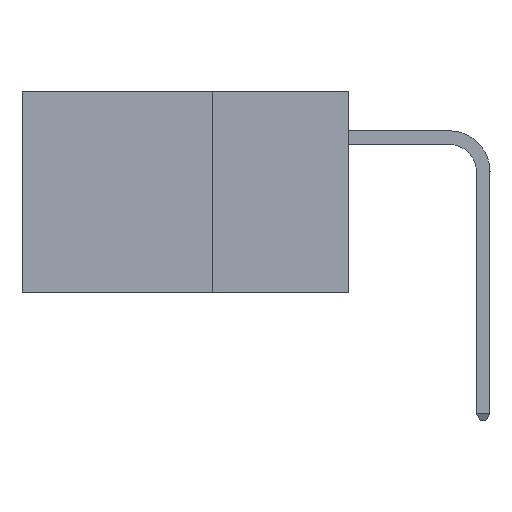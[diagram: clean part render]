
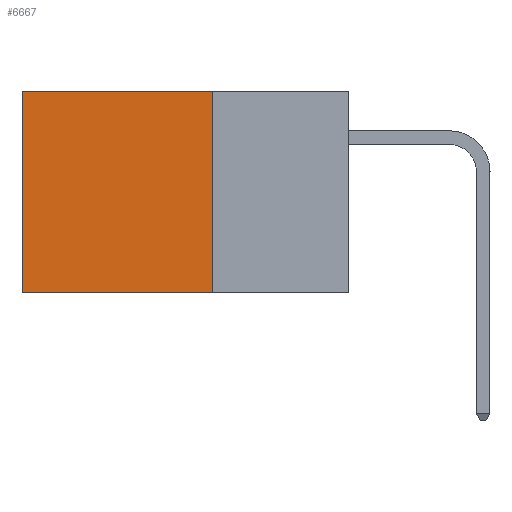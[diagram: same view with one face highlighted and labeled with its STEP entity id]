
A CAD part, left-side view. The second image highlights one B-rep face of the part: STEP entity #6667.
In plain terms, the highlighted planar face has unit normal (-1, 0, 0).
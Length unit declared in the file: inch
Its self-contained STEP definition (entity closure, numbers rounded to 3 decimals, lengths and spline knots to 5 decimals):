
#29 = LINE ( 'NONE', #6393, #11558 ) ;
#331 = VERTEX_POINT ( 'NONE', #14017 ) ;
#605 = VERTEX_POINT ( 'NONE', #11460 ) ;
#2172 = ORIENTED_EDGE ( 'NONE', *, *, #9008, .T. ) ;
#2841 = FACE_OUTER_BOUND ( 'NONE', #14357, .T. ) ;
#3492 = VERTEX_POINT ( 'NONE', #11173 ) ;
#3546 = CARTESIAN_POINT ( 'NONE',  ( 0.2875, 0.6, 0. ) ) ;
#3996 = VERTEX_POINT ( 'NONE', #9984 ) ;
#4261 = VECTOR ( 'NONE', #9499, 39.37008 ) ;
#4561 = VECTOR ( 'NONE', #11154, 39.37008 ) ;
#4612 = LINE ( 'NONE', #8438, #4261 ) ;
#4758 = DIRECTION ( 'NONE',  ( 0., 1., 0. ) ) ;
#5315 = DIRECTION ( 'NONE',  ( 0., 0., -1. ) ) ;
#5615 = VECTOR ( 'NONE', #4758, 39.37008 ) ;
#5926 = CARTESIAN_POINT ( 'NONE',  ( 0.2875, 0.25, -0.37 ) ) ;
#6393 = CARTESIAN_POINT ( 'NONE',  ( 0.2875, 0.25, 0. ) ) ;
#6667 = ADVANCED_FACE ( 'NONE', ( #2841 ), #7517, .F. ) ;
#7362 = AXIS2_PLACEMENT_3D ( 'NONE', #7486, #7462, #7458 ) ;
#7458 = DIRECTION ( 'NONE',  ( 0., 0., -1. ) ) ;
#7462 = DIRECTION ( 'NONE',  ( 1., 0., 0. ) ) ;
#7486 = CARTESIAN_POINT ( 'NONE',  ( 0.2875, 0.25, 0. ) ) ;
#7517 = PLANE ( 'NONE',  #7362 ) ;
#7586 = EDGE_CURVE ( 'NONE', #605, #331, #4612, .T. ) ;
#8438 = CARTESIAN_POINT ( 'NONE',  ( 0.2875, 0.25, 0. ) ) ;
#9008 = EDGE_CURVE ( 'NONE', #331, #3492, #9990, .T. ) ;
#9499 = DIRECTION ( 'NONE',  ( 0., 1., 0. ) ) ;
#9724 = EDGE_CURVE ( 'NONE', #3996, #3492, #11957, .T. ) ;
#9984 = CARTESIAN_POINT ( 'NONE',  ( 0.2875, 0.25, -0.37 ) ) ;
#9990 = LINE ( 'NONE', #3546, #4561 ) ;
#10470 = ORIENTED_EDGE ( 'NONE', *, *, #9724, .F. ) ;
#11154 = DIRECTION ( 'NONE',  ( 0., 0., -1. ) ) ;
#11173 = CARTESIAN_POINT ( 'NONE',  ( 0.2875, 0.6, -0.37 ) ) ;
#11460 = CARTESIAN_POINT ( 'NONE',  ( 0.2875, 0.25, 0. ) ) ;
#11558 = VECTOR ( 'NONE', #5315, 39.37008 ) ;
#11957 = LINE ( 'NONE', #5926, #5615 ) ;
#12267 = EDGE_CURVE ( 'NONE', #605, #3996, #29, .T. ) ;
#12712 = ORIENTED_EDGE ( 'NONE', *, *, #12267, .F. ) ;
#13667 = ORIENTED_EDGE ( 'NONE', *, *, #7586, .T. ) ;
#14017 = CARTESIAN_POINT ( 'NONE',  ( 0.2875, 0.6, 0. ) ) ;
#14357 = EDGE_LOOP ( 'NONE', ( #2172, #10470, #12712, #13667 ) ) ;
